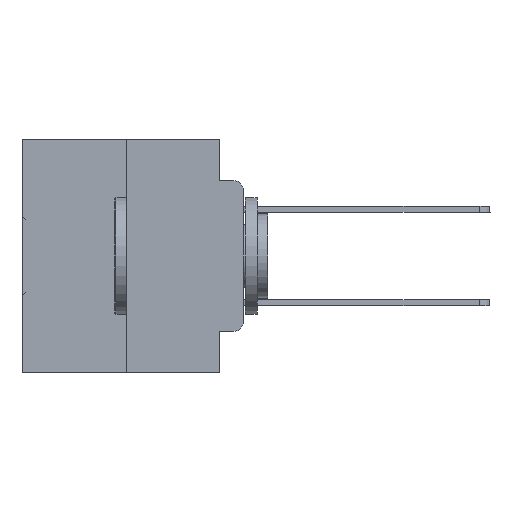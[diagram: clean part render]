
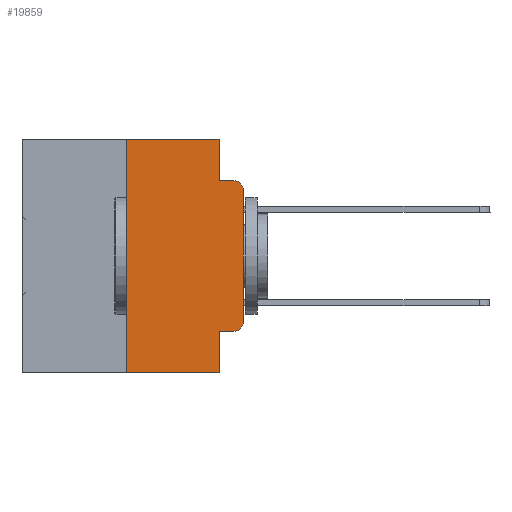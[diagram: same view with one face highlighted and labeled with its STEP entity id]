
A CAD part, left-side view. The second image highlights one B-rep face of the part: STEP entity #19859.
In plain terms, the highlighted planar face has unit normal (-1, 0, 0).
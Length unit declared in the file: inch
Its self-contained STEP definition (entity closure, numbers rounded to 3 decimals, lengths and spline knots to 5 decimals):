
#82 = CARTESIAN_POINT ( 'NONE',  ( 0., 0.051, 0. ) ) ;
#305 = LINE ( 'NONE', #29903, #8714 ) ;
#517 = VERTEX_POINT ( 'NONE', #30096 ) ;
#755 = AXIS2_PLACEMENT_3D ( 'NONE', #18713, #18260, #34569 ) ;
#1835 = CARTESIAN_POINT ( 'NONE',  ( 0., 0.25, 0. ) ) ;
#2601 = DIRECTION ( 'NONE',  ( 0., 0., -1. ) ) ;
#3522 = FACE_OUTER_BOUND ( 'NONE', #26760, .T. ) ;
#3883 = DIRECTION ( 'NONE',  ( 0., 0., -1. ) ) ;
#4710 = EDGE_CURVE ( 'NONE', #8596, #22491, #13438, .T. ) ;
#5002 = DIRECTION ( 'NONE',  ( 0., 0., -1. ) ) ;
#5491 = DIRECTION ( 'NONE',  ( 1., 0., 0. ) ) ;
#5635 = VECTOR ( 'NONE', #29427, 39.37008 ) ;
#5659 = CARTESIAN_POINT ( 'NONE',  ( 0., 0.25, -0.5 ) ) ;
#5916 = LINE ( 'NONE', #27762, #20973 ) ;
#6042 = LINE ( 'NONE', #10730, #5635 ) ;
#6361 = VECTOR ( 'NONE', #30912, 39.37008 ) ;
#6924 = CARTESIAN_POINT ( 'NONE',  ( 0., 0.051, 0. ) ) ;
#7002 = VERTEX_POINT ( 'NONE', #20842 ) ;
#7457 = VECTOR ( 'NONE', #11090, 39.37008 ) ;
#8096 = CARTESIAN_POINT ( 'NONE',  ( 0., 0.02, -0.4115 ) ) ;
#8103 = ORIENTED_EDGE ( 'NONE', *, *, #29832, .T. ) ;
#8596 = VERTEX_POINT ( 'NONE', #5659 ) ;
#8714 = VECTOR ( 'NONE', #29561, 39.37008 ) ;
#10413 = VERTEX_POINT ( 'NONE', #8096 ) ;
#10730 = CARTESIAN_POINT ( 'NONE',  ( 0., 0.473, 0. ) ) ;
#10888 = CARTESIAN_POINT ( 'NONE',  ( 0., 0., 0. ) ) ;
#11040 = EDGE_CURVE ( 'NONE', #23763, #10413, #17898, .T. ) ;
#11090 = DIRECTION ( 'NONE',  ( 0., -1., 0. ) ) ;
#12665 = CARTESIAN_POINT ( 'NONE',  ( 0., 0.25, 0. ) ) ;
#12965 = EDGE_CURVE ( 'NONE', #22491, #24463, #6042, .T. ) ;
#13282 = CARTESIAN_POINT ( 'NONE',  ( 0., 0.051, -0.0885 ) ) ;
#13438 = LINE ( 'NONE', #12665, #6361 ) ;
#13916 = ORIENTED_EDGE ( 'NONE', *, *, #4710, .F. ) ;
#15481 = EDGE_CURVE ( 'NONE', #26416, #7002, #5916, .T. ) ;
#15494 = ORIENTED_EDGE ( 'NONE', *, *, #15481, .F. ) ;
#15840 = CARTESIAN_POINT ( 'NONE',  ( 0., 0.02, -0.1085 ) ) ;
#16208 = CARTESIAN_POINT ( 'NONE',  ( 0., 0.473, -0.5 ) ) ;
#16324 = CARTESIAN_POINT ( 'NONE',  ( 0., 0., -0.3915 ) ) ;
#17553 = ORIENTED_EDGE ( 'NONE', *, *, #11040, .T. ) ;
#17685 = EDGE_CURVE ( 'NONE', #8596, #517, #24542, .T. ) ;
#17898 = LINE ( 'NONE', #17933, #28766 ) ;
#17933 = CARTESIAN_POINT ( 'NONE',  ( 0., 0.051, -0.4115 ) ) ;
#18260 = DIRECTION ( 'NONE',  ( -1., 0., 0. ) ) ;
#18282 = VERTEX_POINT ( 'NONE', #16324 ) ;
#18624 = DIRECTION ( 'NONE',  ( -1., 0., 0. ) ) ;
#18713 = CARTESIAN_POINT ( 'NONE',  ( 0., 0.02, -0.3915 ) ) ;
#18816 = DIRECTION ( 'NONE',  ( 0., 0., 1. ) ) ;
#19859 = ADVANCED_FACE ( 'NONE', ( #3522 ), #34529, .F. ) ;
#20162 = VECTOR ( 'NONE', #3883, 39.37008 ) ;
#20516 = DIRECTION ( 'NONE',  ( 0., -1., 0. ) ) ;
#20842 = CARTESIAN_POINT ( 'NONE',  ( 0., 0.02, -0.0885 ) ) ;
#20973 = VECTOR ( 'NONE', #20516, 39.37008 ) ;
#21653 = CIRCLE ( 'NONE', #755, 0.02 ) ;
#22491 = VERTEX_POINT ( 'NONE', #1835 ) ;
#22687 = EDGE_CURVE ( 'NONE', #10413, #18282, #21653, .T. ) ;
#23192 = EDGE_CURVE ( 'NONE', #27145, #7002, #33694, .T. ) ;
#23347 = VECTOR ( 'NONE', #18816, 39.37008 ) ;
#23763 = VERTEX_POINT ( 'NONE', #28870 ) ;
#24051 = CARTESIAN_POINT ( 'NONE',  ( 0., 0.473, 0. ) ) ;
#24463 = VERTEX_POINT ( 'NONE', #82 ) ;
#24542 = LINE ( 'NONE', #16208, #7457 ) ;
#26084 = EDGE_CURVE ( 'NONE', #24463, #26416, #28111, .T. ) ;
#26262 = LINE ( 'NONE', #10888, #23347 ) ;
#26336 = ORIENTED_EDGE ( 'NONE', *, *, #12965, .F. ) ;
#26416 = VERTEX_POINT ( 'NONE', #13282 ) ;
#26760 = EDGE_LOOP ( 'NONE', ( #8103, #32589, #15494, #27799, #26336, #13916, #32824, #31526, #17553, #30148 ) ) ;
#26938 = AXIS2_PLACEMENT_3D ( 'NONE', #15840, #18624, #5002 ) ;
#27145 = VERTEX_POINT ( 'NONE', #27812 ) ;
#27762 = CARTESIAN_POINT ( 'NONE',  ( 0., 0.051, -0.0885 ) ) ;
#27799 = ORIENTED_EDGE ( 'NONE', *, *, #26084, .F. ) ;
#27812 = CARTESIAN_POINT ( 'NONE',  ( 0., 0., -0.1085 ) ) ;
#28111 = LINE ( 'NONE', #6924, #20162 ) ;
#28766 = VECTOR ( 'NONE', #28799, 39.37008 ) ;
#28799 = DIRECTION ( 'NONE',  ( 0., -1., 0. ) ) ;
#28870 = CARTESIAN_POINT ( 'NONE',  ( 0., 0.051, -0.4115 ) ) ;
#28900 = AXIS2_PLACEMENT_3D ( 'NONE', #24051, #5491, #2601 ) ;
#29427 = DIRECTION ( 'NONE',  ( 0., -1., 0. ) ) ;
#29561 = DIRECTION ( 'NONE',  ( 0., 0., -1. ) ) ;
#29832 = EDGE_CURVE ( 'NONE', #18282, #27145, #26262, .T. ) ;
#29883 = EDGE_CURVE ( 'NONE', #23763, #517, #305, .T. ) ;
#29903 = CARTESIAN_POINT ( 'NONE',  ( 0., 0.051, 0. ) ) ;
#30096 = CARTESIAN_POINT ( 'NONE',  ( 0., 0.051, -0.5 ) ) ;
#30148 = ORIENTED_EDGE ( 'NONE', *, *, #22687, .T. ) ;
#30912 = DIRECTION ( 'NONE',  ( 0., 0., 1. ) ) ;
#31526 = ORIENTED_EDGE ( 'NONE', *, *, #29883, .F. ) ;
#32589 = ORIENTED_EDGE ( 'NONE', *, *, #23192, .T. ) ;
#32824 = ORIENTED_EDGE ( 'NONE', *, *, #17685, .T. ) ;
#33694 = CIRCLE ( 'NONE', #26938, 0.02 ) ;
#34529 = PLANE ( 'NONE',  #28900 ) ;
#34569 = DIRECTION ( 'NONE',  ( 0., 0., -1. ) ) ;
